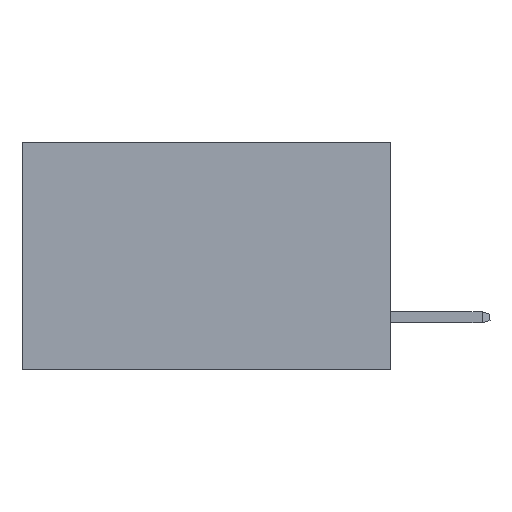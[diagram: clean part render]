
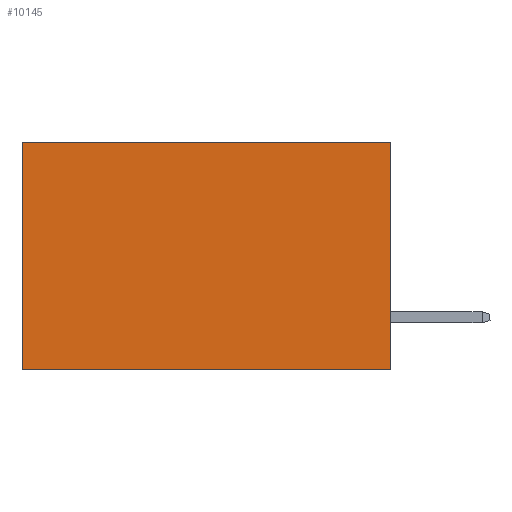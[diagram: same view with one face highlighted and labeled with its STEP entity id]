
A CAD part, left-side view. The second image highlights one B-rep face of the part: STEP entity #10145.
In plain terms, the highlighted planar face has unit normal (-1, 0, 0).
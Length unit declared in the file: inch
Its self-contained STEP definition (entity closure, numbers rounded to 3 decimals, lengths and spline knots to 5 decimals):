
#24 = LINE ( 'NONE', #11806, #3819 ) ;
#106 = CARTESIAN_POINT ( 'NONE',  ( 0.2875, 0., 0. ) ) ;
#1107 = LINE ( 'NONE', #2787, #18216 ) ;
#1408 = VERTEX_POINT ( 'NONE', #19835 ) ;
#1656 = CARTESIAN_POINT ( 'NONE',  ( 0.2875, 0.6, 0. ) ) ;
#2021 = DIRECTION ( 'NONE',  ( 0., 0., -1. ) ) ;
#2703 = EDGE_CURVE ( 'NONE', #18306, #1408, #1107, .T. ) ;
#2787 = CARTESIAN_POINT ( 'NONE',  ( 0.2875, 0., 0. ) ) ;
#2843 = VERTEX_POINT ( 'NONE', #1656 ) ;
#3217 = DIRECTION ( 'NONE',  ( 0., 0., -1. ) ) ;
#3819 = VECTOR ( 'NONE', #13496, 39.37008 ) ;
#3945 = VERTEX_POINT ( 'NONE', #4422 ) ;
#4422 = CARTESIAN_POINT ( 'NONE',  ( 0.2875, 0.6, -0.37 ) ) ;
#5549 = LINE ( 'NONE', #20195, #22042 ) ;
#5966 = EDGE_LOOP ( 'NONE', ( #21502, #12719, #6524, #21592 ) ) ;
#6524 = ORIENTED_EDGE ( 'NONE', *, *, #2703, .F. ) ;
#7652 = DIRECTION ( 'NONE',  ( 0., 0., -1. ) ) ;
#8856 = VECTOR ( 'NONE', #7652, 39.37008 ) ;
#9513 = EDGE_CURVE ( 'NONE', #18306, #2843, #5549, .T. ) ;
#10145 = ADVANCED_FACE ( 'NONE', ( #16697 ), #18935, .F. ) ;
#10267 = DIRECTION ( 'NONE',  ( 0., 1., 0. ) ) ;
#11806 = CARTESIAN_POINT ( 'NONE',  ( 0.2875, 0., -0.37 ) ) ;
#12356 = DIRECTION ( 'NONE',  ( 1., 0., 0. ) ) ;
#12637 = CARTESIAN_POINT ( 'NONE',  ( 0.2875, 0.6, 0. ) ) ;
#12719 = ORIENTED_EDGE ( 'NONE', *, *, #21639, .F. ) ;
#13496 = DIRECTION ( 'NONE',  ( 0., 1., 0. ) ) ;
#14121 = AXIS2_PLACEMENT_3D ( 'NONE', #106, #12356, #2021 ) ;
#16695 = LINE ( 'NONE', #12637, #8856 ) ;
#16697 = FACE_OUTER_BOUND ( 'NONE', #5966, .T. ) ;
#17137 = CARTESIAN_POINT ( 'NONE',  ( 0.2875, 0., 0. ) ) ;
#17150 = EDGE_CURVE ( 'NONE', #2843, #3945, #16695, .T. ) ;
#18216 = VECTOR ( 'NONE', #3217, 39.37008 ) ;
#18306 = VERTEX_POINT ( 'NONE', #17137 ) ;
#18935 = PLANE ( 'NONE',  #14121 ) ;
#19835 = CARTESIAN_POINT ( 'NONE',  ( 0.2875, 0., -0.37 ) ) ;
#20195 = CARTESIAN_POINT ( 'NONE',  ( 0.2875, 0., 0. ) ) ;
#21502 = ORIENTED_EDGE ( 'NONE', *, *, #17150, .T. ) ;
#21592 = ORIENTED_EDGE ( 'NONE', *, *, #9513, .T. ) ;
#21639 = EDGE_CURVE ( 'NONE', #1408, #3945, #24, .T. ) ;
#22042 = VECTOR ( 'NONE', #10267, 39.37008 ) ;
